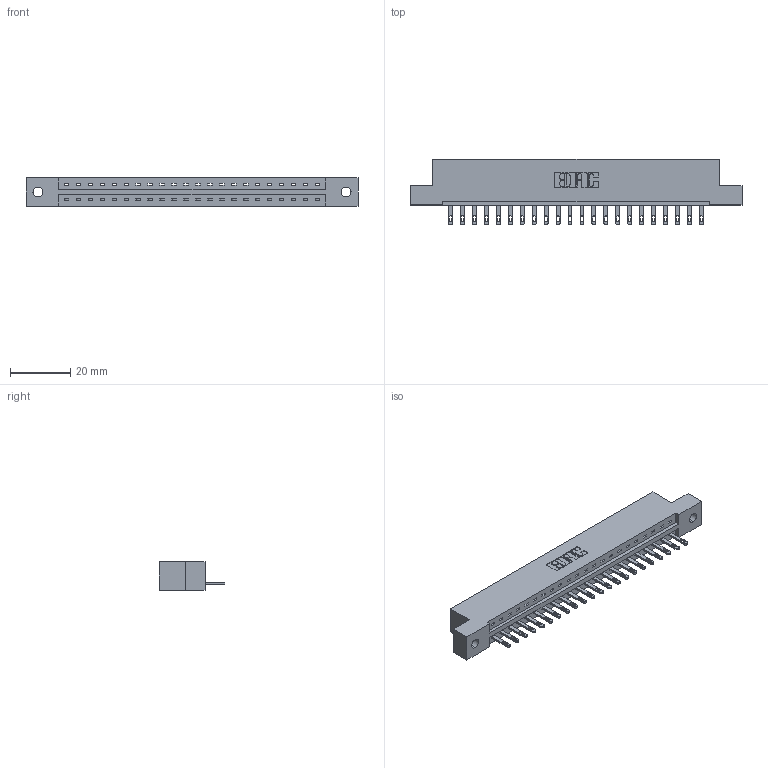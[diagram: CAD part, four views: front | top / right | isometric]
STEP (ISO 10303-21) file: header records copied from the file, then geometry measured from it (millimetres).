
FILE_DESCRIPTION (( 'STEP AP203' ), '1' );
FILE_NAME ('887-022-500-102.STEP', '2020-09-20T18:29:50', ( '' ), ( '' ), 'SwSTEP 2.0', 'SolidWorks 2020', '' );
FILE_SCHEMA (( 'CONFIG_CONTROL_DESIGN' ));
Length unit declared in the file: inch
Products named in the file (3): 345-292-001_345-293-100; 887-022-500-102; 837 Part_Flush Mounting Lugs - 0.128 Dia
Assembly tree (23 placements, depth 2):
  887-022-500-102
    837 Part_Flush Mounting Lugs - 0.128 Dia
    345-292-001_345-293-100  x22
Bounding box: 110.19 x 21.85 x 9.4 mm (x, y, z)
Volume: 11178.6 mm3; surface area: 11221.9 mm2
Topology: 23 solids, 23 shells, 1390 faces, 4271 edges, 2846 vertices
Faces by surface type: plane 950, cylinder 440
Entity records: 18873 total; most frequent: CARTESIAN_POINT 3292, ORIENTED_EDGE 3250, DIRECTION 2813, EDGE_CURVE 1625, VECTOR 1493, LINE 1493, VERTEX_POINT 1082, AXIS2_PLACEMENT_3D 660
